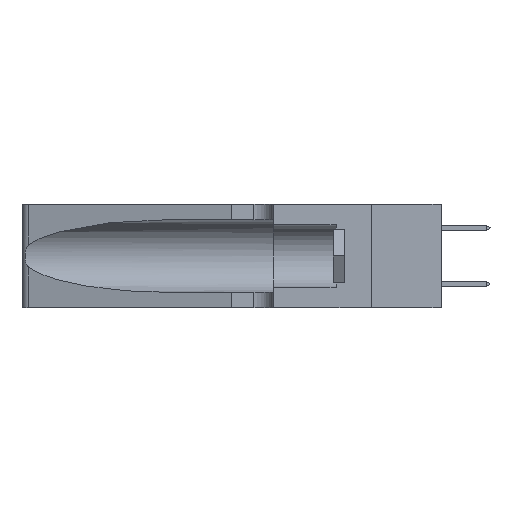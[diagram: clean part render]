
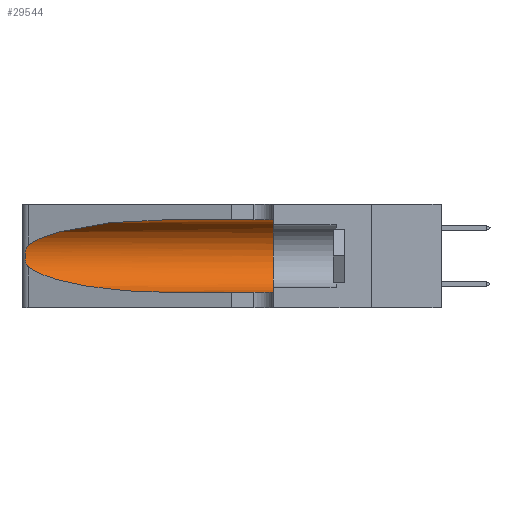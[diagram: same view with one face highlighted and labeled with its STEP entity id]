
A CAD part, left-side view. The second image highlights one B-rep face of the part: STEP entity #29544.
In plain terms, the highlighted cylindrical face has radius 3.308 mm (diameter 6.617 mm), a partial arc.
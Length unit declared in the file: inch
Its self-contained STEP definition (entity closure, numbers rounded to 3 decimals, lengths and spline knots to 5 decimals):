
#233 = CARTESIAN_POINT ( 'NONE',  ( 0.25487, 1.22718, 0.14631 ) ) ;
#1887 = VECTOR ( 'NONE', #22075, 39.37008 ) ;
#2045 = CARTESIAN_POINT ( 'NONE',  ( 0.25487, 1.22718, 0.22369 ) ) ;
#3196 = AXIS2_PLACEMENT_3D ( 'NONE', #28988, #37697, #32105 ) ;
#3645 = EDGE_CURVE ( 'NONE', #10893, #6362, #24282, .T. ) ;
#3665 = AXIS2_PLACEMENT_3D ( 'NONE', #24023, #23900, #5571 ) ;
#4821 = CARTESIAN_POINT ( 'NONE',  ( 0.26075, 1.23896, 0.178 ) ) ;
#5067 = CIRCLE ( 'NONE', #3665, 0.13025 ) ;
#5367 = CARTESIAN_POINT ( 'NONE',  ( 0.25555, 1.22993, 0.14849 ) ) ;
#5571 = DIRECTION ( 'NONE',  ( 0., 0., 1. ) ) ;
#5615 = CARTESIAN_POINT ( 'NONE',  ( 0.18966, 0.96281, 0.31525 ) ) ;
#5812 = FACE_OUTER_BOUND ( 'NONE', #37606, .T. ) ;
#6362 = VERTEX_POINT ( 'NONE', #18176 ) ;
#6609 = VERTEX_POINT ( 'NONE', #36609 ) ;
#7683 = CARTESIAN_POINT ( 'NONE',  ( 0.25787, 1.23484, 0.2124 ) ) ;
#7952 = CARTESIAN_POINT ( 'NONE',  ( 0.25555, 1.22994, 0.2215 ) ) ;
#8020 = ORIENTED_EDGE ( 'NONE', *, *, #12668, .T. ) ;
#8072 = CARTESIAN_POINT ( 'NONE',  ( 0.26018, 1.23835, 0.19895 ) ) ;
#8216 = B_SPLINE_CURVE_WITH_KNOTS ( 'NONE', 3,
 ( #2045, #7952, #38332, #7683, #38609, #8072, #10784, #4821, #26376, #11041, #17203, #23703, #5367, #23967 ),
 .UNSPECIFIED., .F., .F.,
 ( 4, 2, 2, 2, 2, 2, 4 ),
 ( 0., 0.00027, 0.00053, 0.00107, 0.0016, 0.00187, 0.00214 ),
 .UNSPECIFIED. ) ;
#8232 = CARTESIAN_POINT ( 'NONE',  ( 0.1305, 0.35, 0.31525 ) ) ;
#8448 = CARTESIAN_POINT ( 'NONE',  ( 0.1305, 0.72297, 0.31525 ) ) ;
#9872 = VERTEX_POINT ( 'NONE', #27453 ) ;
#10784 = CARTESIAN_POINT ( 'NONE',  ( 0.26075, 1.23896, 0.19203 ) ) ;
#10893 = VERTEX_POINT ( 'NONE', #8448 ) ;
#11041 = CARTESIAN_POINT ( 'NONE',  ( 0.25856, 1.23593, 0.16098 ) ) ;
#11330 = EDGE_CURVE ( 'NONE', #14378, #9872, #5067, .T. ) ;
#11997 = ORIENTED_EDGE ( 'NONE', *, *, #20656, .T. ) ;
#12287 = DIRECTION ( 'NONE',  ( 0., -1., 0. ) ) ;
#12668 = EDGE_CURVE ( 'NONE', #6362, #25161, #8216, .T. ) ;
#12927 = CARTESIAN_POINT ( 'NONE',  ( 0.18966, 0.96281, 0.05475 ) ) ;
#14378 = VERTEX_POINT ( 'NONE', #8232 ) ;
#15794 = LINE ( 'NONE', #18069, #1887 ) ;
#17203 = CARTESIAN_POINT ( 'NONE',  ( 0.25789, 1.23486, 0.15765 ) ) ;
#18069 = CARTESIAN_POINT ( 'NONE',  ( 0.1305, 1.61858, 0.05475 ) ) ;
#18093 = CARTESIAN_POINT ( 'NONE',  ( 0.1305, 1.61858, 0.31525 ) ) ;
#18176 = CARTESIAN_POINT ( 'NONE',  ( 0.25487, 1.22718, 0.22369 ) ) ;
#19371 = EDGE_CURVE ( 'NONE', #10893, #14378, #35663, .T. ) ;
#20087 = ORIENTED_EDGE ( 'NONE', *, *, #3645, .T. ) ;
#20264 = CYLINDRICAL_SURFACE ( 'NONE', #3196, 0.13025 ) ;
#20656 = EDGE_CURVE ( 'NONE', #6609, #9872, #15794, .T. ) ;
#20927 = ORIENTED_EDGE ( 'NONE', *, *, #25959, .T. ) ;
#22075 = DIRECTION ( 'NONE',  ( 0., -1., 0. ) ) ;
#23703 = CARTESIAN_POINT ( 'NONE',  ( 0.25639, 1.23186, 0.15144 ) ) ;
#23749 = ORIENTED_EDGE ( 'NONE', *, *, #19371, .F. ) ;
#23900 = DIRECTION ( 'NONE',  ( 0., 1., 0. ) ) ;
#23967 = CARTESIAN_POINT ( 'NONE',  ( 0.25487, 1.22718, 0.14631 ) ) ;
#24023 = CARTESIAN_POINT ( 'NONE',  ( 0.1305, 0.35, 0.185 ) ) ;
#24282 =( BOUNDED_CURVE ( )  B_SPLINE_CURVE ( 3, ( #33623, #5615, #33363, #27283 ),
 .UNSPECIFIED., .F., .F. ) 
 B_SPLINE_CURVE_WITH_KNOTS ( ( 4, 4 ),
 ( 1.5708, 2.84003 ),
 .UNSPECIFIED. ) 
 CURVE ( )  GEOMETRIC_REPRESENTATION_ITEM ( )  RATIONAL_B_SPLINE_CURVE ( ( 1., 0.87, 0.87, 1. ) ) 
 REPRESENTATION_ITEM ( '' )  );
#24503 =( BOUNDED_CURVE ( )  B_SPLINE_CURVE ( 3, ( #37030, #37281, #12927, #38223 ),
 .UNSPECIFIED., .F., .F. ) 
 B_SPLINE_CURVE_WITH_KNOTS ( ( 4, 4 ),
 ( 3.44316, 4.71239 ),
 .UNSPECIFIED. ) 
 CURVE ( )  GEOMETRIC_REPRESENTATION_ITEM ( )  RATIONAL_B_SPLINE_CURVE ( ( 1., 0.87, 0.87, 1. ) ) 
 REPRESENTATION_ITEM ( '' )  );
#25161 = VERTEX_POINT ( 'NONE', #233 ) ;
#25959 = EDGE_CURVE ( 'NONE', #25161, #6609, #24503, .T. ) ;
#26046 = VECTOR ( 'NONE', #12287, 39.37008 ) ;
#26376 = CARTESIAN_POINT ( 'NONE',  ( 0.26017, 1.23833, 0.17102 ) ) ;
#27283 = CARTESIAN_POINT ( 'NONE',  ( 0.25487, 1.22718, 0.22369 ) ) ;
#27453 = CARTESIAN_POINT ( 'NONE',  ( 0.1305, 0.35, 0.05475 ) ) ;
#28988 = CARTESIAN_POINT ( 'NONE',  ( 0.1305, 1.61858, 0.185 ) ) ;
#29544 = ADVANCED_FACE ( 'NONE', ( #5812 ), #20264, .F. ) ;
#32105 = DIRECTION ( 'NONE',  ( 0., 0., -1. ) ) ;
#33363 = CARTESIAN_POINT ( 'NONE',  ( 0.2373, 1.15595, 0.28018 ) ) ;
#33623 = CARTESIAN_POINT ( 'NONE',  ( 0.1305, 0.72297, 0.31525 ) ) ;
#35663 = LINE ( 'NONE', #18093, #26046 ) ;
#36609 = CARTESIAN_POINT ( 'NONE',  ( 0.1305, 0.72297, 0.05475 ) ) ;
#37030 = CARTESIAN_POINT ( 'NONE',  ( 0.25487, 1.22718, 0.14631 ) ) ;
#37281 = CARTESIAN_POINT ( 'NONE',  ( 0.2373, 1.15595, 0.08982 ) ) ;
#37606 = EDGE_LOOP ( 'NONE', ( #20087, #8020, #20927, #11997, #37655, #23749 ) ) ;
#37655 = ORIENTED_EDGE ( 'NONE', *, *, #11330, .F. ) ;
#37697 = DIRECTION ( 'NONE',  ( 0., -1., 0. ) ) ;
#38223 = CARTESIAN_POINT ( 'NONE',  ( 0.1305, 0.72297, 0.05475 ) ) ;
#38332 = CARTESIAN_POINT ( 'NONE',  ( 0.25639, 1.23184, 0.21858 ) ) ;
#38609 = CARTESIAN_POINT ( 'NONE',  ( 0.25854, 1.2359, 0.20912 ) ) ;
